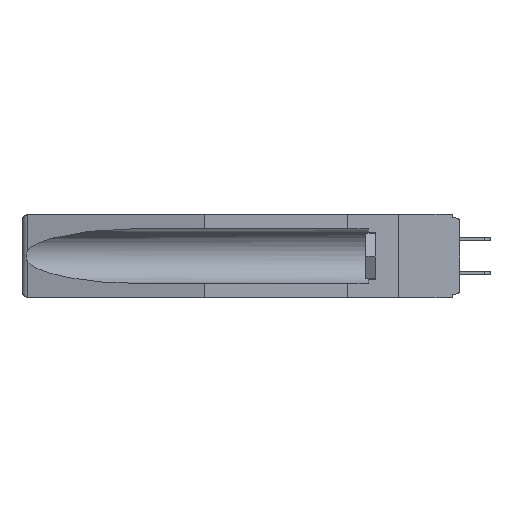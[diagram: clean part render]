
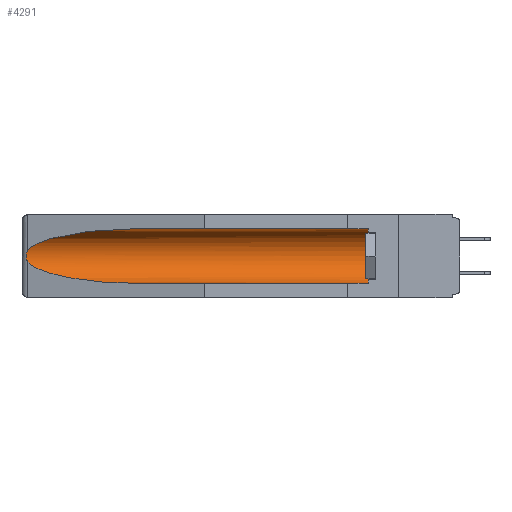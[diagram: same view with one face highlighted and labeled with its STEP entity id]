
A CAD part, left-side view. The second image highlights one B-rep face of the part: STEP entity #4291.
In plain terms, the highlighted cylindrical face has radius 2.857 mm (diameter 5.715 mm), a partial arc.
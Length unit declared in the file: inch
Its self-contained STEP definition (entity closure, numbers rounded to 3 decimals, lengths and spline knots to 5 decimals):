
#499 = CARTESIAN_POINT ( 'NONE',  ( 0.26597, 1.5296, -0.19026 ) ) ;
#729 = VERTEX_POINT ( 'NONE', #9704 ) ;
#1204 = B_SPLINE_CURVE_WITH_KNOTS ( 'NONE', 3,
 ( #6519, #11206, #18813, #17420, #8213, #12877, #9630, #12813, #499, #3631 ),
 .UNSPECIFIED., .F., .F.,
 ( 4, 2, 2, 2, 4 ),
 ( 0., 0.00029, 0.00058, 0.00087, 0.00117 ),
 .UNSPECIFIED. ) ;
#1805 = VERTEX_POINT ( 'NONE', #1844 ) ;
#1844 = CARTESIAN_POINT ( 'NONE',  ( 0.26537, 1.52718, -0.19328 ) ) ;
#2430 = VECTOR ( 'NONE', #2525, 39.37008 ) ;
#2525 = DIRECTION ( 'NONE',  ( 0., 1., 0. ) ) ;
#3003 = FACE_OUTER_BOUND ( 'NONE', #7346, .T. ) ;
#3077 = LINE ( 'NONE', #8871, #5517 ) ;
#3184 = ORIENTED_EDGE ( 'NONE', *, *, #7577, .F. ) ;
#3377 = LINE ( 'NONE', #9808, #2430 ) ;
#3631 = CARTESIAN_POINT ( 'NONE',  ( 0.26537, 1.52718, -0.19328 ) ) ;
#4291 = ADVANCED_FACE ( 'NONE', ( #3003 ), #16004, .F. ) ;
#4327 = CARTESIAN_POINT ( 'NONE',  ( 0.155, 1.07973, -0.284 ) ) ;
#4351 = VERTEX_POINT ( 'NONE', #17992 ) ;
#5517 = VECTOR ( 'NONE', #16671, 39.37008 ) ;
#5905 = EDGE_CURVE ( 'NONE', #1805, #6997, #8374, .T. ) ;
#5918 = DIRECTION ( 'NONE',  ( 0., -1., 0. ) ) ;
#6519 = CARTESIAN_POINT ( 'NONE',  ( 0.26537, 1.52718, -0.14972 ) ) ;
#6997 = VERTEX_POINT ( 'NONE', #4327 ) ;
#7322 = CARTESIAN_POINT ( 'NONE',  ( 0.25451, 1.48313, -0.24835 ) ) ;
#7346 = EDGE_LOOP ( 'NONE', ( #15907, #16335, #10641, #3184, #12912, #17595 ) ) ;
#7458 = CARTESIAN_POINT ( 'NONE',  ( 0.26537, 1.52718, -0.19328 ) ) ;
#7577 = EDGE_CURVE ( 'NONE', #15195, #6997, #3377, .T. ) ;
#8213 = CARTESIAN_POINT ( 'NONE',  ( 0.2675, 1.53308, -0.16763 ) ) ;
#8374 =( BOUNDED_CURVE ( )  B_SPLINE_CURVE ( 3, ( #7458, #7322, #13618, #8966 ),
 .UNSPECIFIED., .F., .F. ) 
 B_SPLINE_CURVE_WITH_KNOTS ( ( 4, 4 ),
 ( 0.1948, 1.5708 ),
 .UNSPECIFIED. ) 
 CURVE ( )  GEOMETRIC_REPRESENTATION_ITEM ( )  RATIONAL_B_SPLINE_CURVE ( ( 1., 0.848, 0.848, 1. ) ) 
 REPRESENTATION_ITEM ( '' )  );
#8388 = CARTESIAN_POINT ( 'NONE',  ( 0.155, -0.30754, -0.1715 ) ) ;
#8871 = CARTESIAN_POINT ( 'NONE',  ( 0.155, -0.30754, -0.059 ) ) ;
#8966 = CARTESIAN_POINT ( 'NONE',  ( 0.155, 1.07973, -0.284 ) ) ;
#9630 = CARTESIAN_POINT ( 'NONE',  ( 0.2673, 1.53269, -0.17917 ) ) ;
#9704 = CARTESIAN_POINT ( 'NONE',  ( 0.26537, 1.52718, -0.14972 ) ) ;
#9808 = CARTESIAN_POINT ( 'NONE',  ( 0.155, -0.30754, -0.284 ) ) ;
#10557 = AXIS2_PLACEMENT_3D ( 'NONE', #8388, #11451, #14462 ) ;
#10641 = ORIENTED_EDGE ( 'NONE', *, *, #5905, .T. ) ;
#10749 = EDGE_CURVE ( 'NONE', #15195, #4351, #13709, .T. ) ;
#10856 = CARTESIAN_POINT ( 'NONE',  ( 0.26537, 1.52718, -0.14972 ) ) ;
#11026 = AXIS2_PLACEMENT_3D ( 'NONE', #16737, #5918, #18084 ) ;
#11206 = CARTESIAN_POINT ( 'NONE',  ( 0.26597, 1.52961, -0.15275 ) ) ;
#11451 = DIRECTION ( 'NONE',  ( 0., 1., 0. ) ) ;
#11464 = VERTEX_POINT ( 'NONE', #15402 ) ;
#12253 = CARTESIAN_POINT ( 'NONE',  ( 0.21114, 1.30732, -0.059 ) ) ;
#12472 = CARTESIAN_POINT ( 'NONE',  ( 0.155, 0.126, -0.284 ) ) ;
#12813 = CARTESIAN_POINT ( 'NONE',  ( 0.26655, 1.53094, -0.18657 ) ) ;
#12877 = CARTESIAN_POINT ( 'NONE',  ( 0.2675, 1.53308, -0.17534 ) ) ;
#12912 = ORIENTED_EDGE ( 'NONE', *, *, #10749, .T. ) ;
#13179 = EDGE_CURVE ( 'NONE', #4351, #11464, #3077, .T. ) ;
#13618 = CARTESIAN_POINT ( 'NONE',  ( 0.21114, 1.30732, -0.284 ) ) ;
#13709 = CIRCLE ( 'NONE', #11026, 0.1125 ) ;
#13995 = CARTESIAN_POINT ( 'NONE',  ( 0.155, 1.07973, -0.059 ) ) ;
#14462 = DIRECTION ( 'NONE',  ( 0., 0., 1. ) ) ;
#14863 = EDGE_CURVE ( 'NONE', #11464, #729, #16123, .T. ) ;
#15195 = VERTEX_POINT ( 'NONE', #12472 ) ;
#15402 = CARTESIAN_POINT ( 'NONE',  ( 0.155, 1.07973, -0.059 ) ) ;
#15907 = ORIENTED_EDGE ( 'NONE', *, *, #14863, .T. ) ;
#16004 = CYLINDRICAL_SURFACE ( 'NONE', #10557, 0.1125 ) ;
#16123 =( BOUNDED_CURVE ( )  B_SPLINE_CURVE ( 3, ( #13995, #12253, #18473, #10856 ),
 .UNSPECIFIED., .F., .F. ) 
 B_SPLINE_CURVE_WITH_KNOTS ( ( 4, 4 ),
 ( 4.71239, 6.08839 ),
 .UNSPECIFIED. ) 
 CURVE ( )  GEOMETRIC_REPRESENTATION_ITEM ( )  RATIONAL_B_SPLINE_CURVE ( ( 1., 0.848, 0.848, 1. ) ) 
 REPRESENTATION_ITEM ( '' )  );
#16335 = ORIENTED_EDGE ( 'NONE', *, *, #17178, .T. ) ;
#16671 = DIRECTION ( 'NONE',  ( 0., 1., 0. ) ) ;
#16737 = CARTESIAN_POINT ( 'NONE',  ( 0.155, 0.126, -0.1715 ) ) ;
#17178 = EDGE_CURVE ( 'NONE', #729, #1805, #1204, .T. ) ;
#17420 = CARTESIAN_POINT ( 'NONE',  ( 0.2673, 1.5327, -0.16383 ) ) ;
#17595 = ORIENTED_EDGE ( 'NONE', *, *, #13179, .T. ) ;
#17992 = CARTESIAN_POINT ( 'NONE',  ( 0.155, 0.126, -0.059 ) ) ;
#18084 = DIRECTION ( 'NONE',  ( 0., 0., 1. ) ) ;
#18473 = CARTESIAN_POINT ( 'NONE',  ( 0.25451, 1.48313, -0.09465 ) ) ;
#18813 = CARTESIAN_POINT ( 'NONE',  ( 0.26654, 1.53092, -0.15636 ) ) ;
